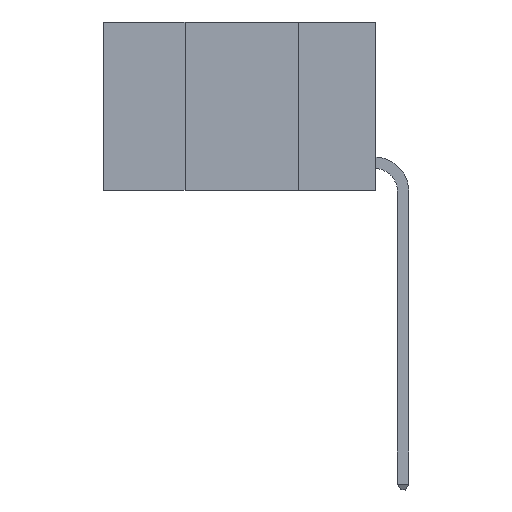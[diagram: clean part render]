
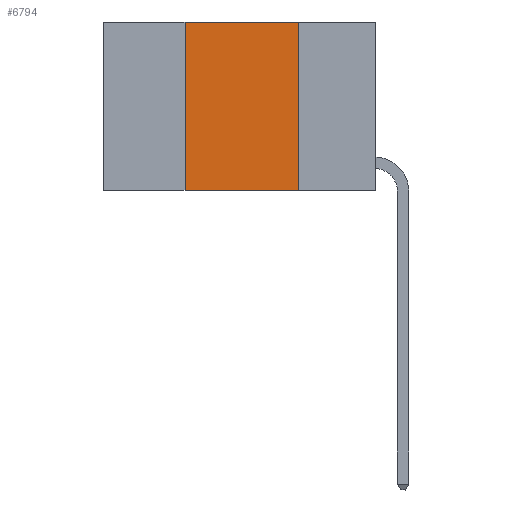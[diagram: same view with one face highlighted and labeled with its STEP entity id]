
A CAD part, left-side view. The second image highlights one B-rep face of the part: STEP entity #6794.
In plain terms, the highlighted planar face has unit normal (-1, 0, 0).
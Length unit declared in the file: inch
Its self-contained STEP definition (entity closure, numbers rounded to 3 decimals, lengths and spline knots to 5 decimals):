
#30 = VERTEX_POINT ( 'NONE', #4941 ) ;
#874 = EDGE_CURVE ( 'NONE', #3537, #6665, #5687, .T. ) ;
#1765 = VECTOR ( 'NONE', #7570, 39.37008 ) ;
#2500 = AXIS2_PLACEMENT_3D ( 'NONE', #3276, #13291, #4766 ) ;
#2752 = CARTESIAN_POINT ( 'NONE',  ( 0., 0.6, 0. ) ) ;
#3168 = CARTESIAN_POINT ( 'NONE',  ( 0., 0.17, 0. ) ) ;
#3276 = CARTESIAN_POINT ( 'NONE',  ( 0., 0.6, 0. ) ) ;
#3537 = VERTEX_POINT ( 'NONE', #4955 ) ;
#4253 = VERTEX_POINT ( 'NONE', #14700 ) ;
#4337 = LINE ( 'NONE', #11166, #15261 ) ;
#4703 = PLANE ( 'NONE',  #2500 ) ;
#4766 = DIRECTION ( 'NONE',  ( 0., 0., -1. ) ) ;
#4941 = CARTESIAN_POINT ( 'NONE',  ( 0., 0.42, -0.37 ) ) ;
#4955 = CARTESIAN_POINT ( 'NONE',  ( 0., 0.17, 0. ) ) ;
#4978 = LINE ( 'NONE', #5470, #12090 ) ;
#5470 = CARTESIAN_POINT ( 'NONE',  ( 0., 0.42, 0. ) ) ;
#5687 = LINE ( 'NONE', #3168, #1765 ) ;
#6665 = VERTEX_POINT ( 'NONE', #17156 ) ;
#6794 = ADVANCED_FACE ( 'NONE', ( #9893 ), #4703, .F. ) ;
#6962 = LINE ( 'NONE', #2752, #18230 ) ;
#7088 = EDGE_CURVE ( 'NONE', #30, #4253, #4978, .T. ) ;
#7341 = ORIENTED_EDGE ( 'NONE', *, *, #7088, .F. ) ;
#7570 = DIRECTION ( 'NONE',  ( 0., 0., -1. ) ) ;
#9498 = ORIENTED_EDGE ( 'NONE', *, *, #874, .F. ) ;
#9893 = FACE_OUTER_BOUND ( 'NONE', #10516, .T. ) ;
#10516 = EDGE_LOOP ( 'NONE', ( #9498, #18461, #7341, #18003 ) ) ;
#10907 = EDGE_CURVE ( 'NONE', #30, #6665, #4337, .T. ) ;
#11166 = CARTESIAN_POINT ( 'NONE',  ( 0., 0.6, -0.37 ) ) ;
#12090 = VECTOR ( 'NONE', #18142, 39.37008 ) ;
#12784 = DIRECTION ( 'NONE',  ( 0., -1., 0. ) ) ;
#13291 = DIRECTION ( 'NONE',  ( 1., 0., 0. ) ) ;
#14700 = CARTESIAN_POINT ( 'NONE',  ( 0., 0.42, 0. ) ) ;
#15261 = VECTOR ( 'NONE', #18179, 39.37008 ) ;
#16470 = EDGE_CURVE ( 'NONE', #4253, #3537, #6962, .T. ) ;
#17156 = CARTESIAN_POINT ( 'NONE',  ( 0., 0.17, -0.37 ) ) ;
#18003 = ORIENTED_EDGE ( 'NONE', *, *, #10907, .T. ) ;
#18142 = DIRECTION ( 'NONE',  ( 0., 0., 1. ) ) ;
#18179 = DIRECTION ( 'NONE',  ( 0., -1., 0. ) ) ;
#18230 = VECTOR ( 'NONE', #12784, 39.37008 ) ;
#18461 = ORIENTED_EDGE ( 'NONE', *, *, #16470, .F. ) ;
